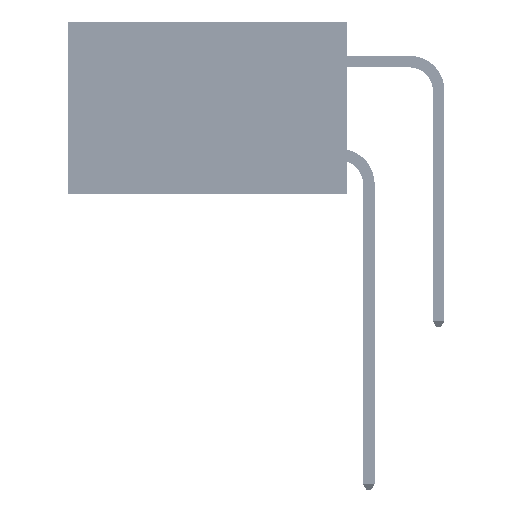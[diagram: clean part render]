
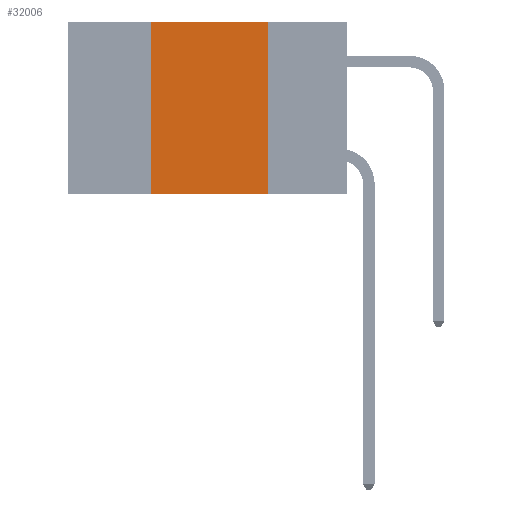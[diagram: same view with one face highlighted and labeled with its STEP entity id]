
A CAD part, left-side view. The second image highlights one B-rep face of the part: STEP entity #32006.
In plain terms, the highlighted planar face has unit normal (-1, 0, 0).
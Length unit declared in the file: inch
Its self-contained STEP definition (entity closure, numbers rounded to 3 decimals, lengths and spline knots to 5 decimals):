
#1905 = VERTEX_POINT ( 'NONE', #31384 ) ;
#5442 = LINE ( 'NONE', #15767, #14294 ) ;
#7149 = ORIENTED_EDGE ( 'NONE', *, *, #44739, .F. ) ;
#10001 = DIRECTION ( 'NONE',  ( 1., 0., 0. ) ) ;
#10183 = LINE ( 'NONE', #33653, #39156 ) ;
#10597 = EDGE_CURVE ( 'NONE', #29488, #39395, #37601, .T. ) ;
#10897 = CARTESIAN_POINT ( 'NONE',  ( 0., 0.17, -0.37 ) ) ;
#11834 = ORIENTED_EDGE ( 'NONE', *, *, #10597, .F. ) ;
#12200 = DIRECTION ( 'NONE',  ( 0., -1., 0. ) ) ;
#12484 = DIRECTION ( 'NONE',  ( 0., 0., -1. ) ) ;
#14294 = VECTOR ( 'NONE', #15941, 39.37008 ) ;
#14965 = CARTESIAN_POINT ( 'NONE',  ( 0., 0.42, 0. ) ) ;
#15767 = CARTESIAN_POINT ( 'NONE',  ( 0., 0.6, -0.37 ) ) ;
#15778 = EDGE_CURVE ( 'NONE', #1905, #38085, #10183, .T. ) ;
#15941 = DIRECTION ( 'NONE',  ( 0., -1., 0. ) ) ;
#16877 = CARTESIAN_POINT ( 'NONE',  ( 0., 0.17, 0. ) ) ;
#21525 = AXIS2_PLACEMENT_3D ( 'NONE', #47630, #10001, #36413 ) ;
#23303 = CARTESIAN_POINT ( 'NONE',  ( 0., 0.6, 0. ) ) ;
#23560 = FACE_OUTER_BOUND ( 'NONE', #46420, .T. ) ;
#29488 = VERTEX_POINT ( 'NONE', #16877 ) ;
#31384 = CARTESIAN_POINT ( 'NONE',  ( 0., 0.42, -0.37 ) ) ;
#32006 = ADVANCED_FACE ( 'NONE', ( #23560 ), #32618, .F. ) ;
#32618 = PLANE ( 'NONE',  #21525 ) ;
#33653 = CARTESIAN_POINT ( 'NONE',  ( 0., 0.42, 0. ) ) ;
#34363 = ORIENTED_EDGE ( 'NONE', *, *, #45483, .T. ) ;
#36413 = DIRECTION ( 'NONE',  ( 0., 0., -1. ) ) ;
#36734 = LINE ( 'NONE', #23303, #45582 ) ;
#37474 = DIRECTION ( 'NONE',  ( 0., 0., 1. ) ) ;
#37601 = LINE ( 'NONE', #42694, #47636 ) ;
#38085 = VERTEX_POINT ( 'NONE', #14965 ) ;
#39156 = VECTOR ( 'NONE', #37474, 39.37008 ) ;
#39395 = VERTEX_POINT ( 'NONE', #10897 ) ;
#42614 = ORIENTED_EDGE ( 'NONE', *, *, #15778, .F. ) ;
#42694 = CARTESIAN_POINT ( 'NONE',  ( 0., 0.17, 0. ) ) ;
#44739 = EDGE_CURVE ( 'NONE', #38085, #29488, #36734, .T. ) ;
#45483 = EDGE_CURVE ( 'NONE', #1905, #39395, #5442, .T. ) ;
#45582 = VECTOR ( 'NONE', #12200, 39.37008 ) ;
#46420 = EDGE_LOOP ( 'NONE', ( #11834, #7149, #42614, #34363 ) ) ;
#47630 = CARTESIAN_POINT ( 'NONE',  ( 0., 0.6, 0. ) ) ;
#47636 = VECTOR ( 'NONE', #12484, 39.37008 ) ;
